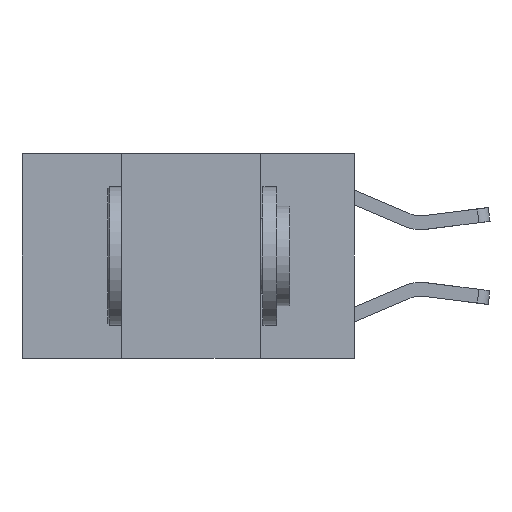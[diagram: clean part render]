
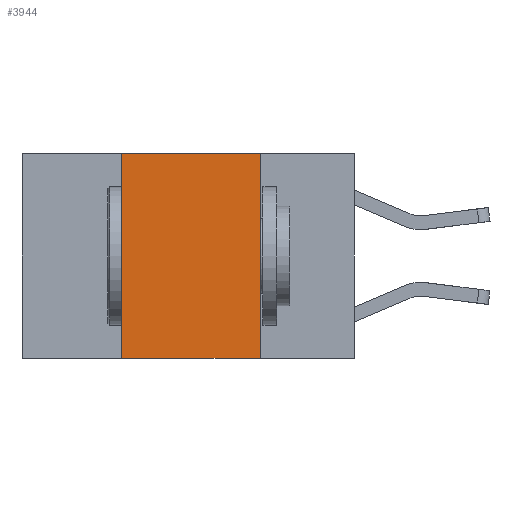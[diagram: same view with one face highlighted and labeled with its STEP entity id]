
A CAD part, left-side view. The second image highlights one B-rep face of the part: STEP entity #3944.
In plain terms, the highlighted planar face has unit normal (-1, 0, 0).
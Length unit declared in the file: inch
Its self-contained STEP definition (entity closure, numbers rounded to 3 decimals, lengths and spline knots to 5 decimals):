
#941 = AXIS2_PLACEMENT_3D ( 'NONE', #8948, #4340, #2792 ) ;
#1291 = ORIENTED_EDGE ( 'NONE', *, *, #2422, .F. ) ;
#1831 = DIRECTION ( 'NONE',  ( 0., 0., -1. ) ) ;
#1952 = ORIENTED_EDGE ( 'NONE', *, *, #6534, .F. ) ;
#2422 = EDGE_CURVE ( 'NONE', #3168, #3902, #9330, .T. ) ;
#2683 = VECTOR ( 'NONE', #4511, 39.37008 ) ;
#2792 = DIRECTION ( 'NONE',  ( 0., 0., -1. ) ) ;
#3014 = CARTESIAN_POINT ( 'NONE',  ( 0., 0.6, 0. ) ) ;
#3054 = LINE ( 'NONE', #8457, #4012 ) ;
#3105 = DIRECTION ( 'NONE',  ( 0., -1., 0. ) ) ;
#3168 = VERTEX_POINT ( 'NONE', #9016 ) ;
#3564 = VECTOR ( 'NONE', #4637, 39.37008 ) ;
#3902 = VERTEX_POINT ( 'NONE', #9345 ) ;
#3944 = ADVANCED_FACE ( 'NONE', ( #5089 ), #9685, .F. ) ;
#4012 = VECTOR ( 'NONE', #3105, 39.37008 ) ;
#4340 = DIRECTION ( 'NONE',  ( 1., 0., 0. ) ) ;
#4456 = VERTEX_POINT ( 'NONE', #6761 ) ;
#4511 = DIRECTION ( 'NONE',  ( 0., -1., 0. ) ) ;
#4637 = DIRECTION ( 'NONE',  ( 0., 0., 1. ) ) ;
#4737 = CARTESIAN_POINT ( 'NONE',  ( 0., 0.42, 0. ) ) ;
#4993 = EDGE_CURVE ( 'NONE', #3168, #7011, #3054, .T. ) ;
#5089 = FACE_OUTER_BOUND ( 'NONE', #5743, .T. ) ;
#5211 = ORIENTED_EDGE ( 'NONE', *, *, #9650, .F. ) ;
#5688 = CARTESIAN_POINT ( 'NONE',  ( 0., 0.17, 0. ) ) ;
#5743 = EDGE_LOOP ( 'NONE', ( #5211, #1952, #1291, #8665 ) ) ;
#6534 = EDGE_CURVE ( 'NONE', #3902, #4456, #9758, .T. ) ;
#6761 = CARTESIAN_POINT ( 'NONE',  ( 0., 0.17, 0. ) ) ;
#7011 = VERTEX_POINT ( 'NONE', #7456 ) ;
#7028 = VECTOR ( 'NONE', #1831, 39.37008 ) ;
#7456 = CARTESIAN_POINT ( 'NONE',  ( 0., 0.17, -0.37 ) ) ;
#7770 = LINE ( 'NONE', #5688, #7028 ) ;
#8457 = CARTESIAN_POINT ( 'NONE',  ( 0., 0.6, -0.37 ) ) ;
#8665 = ORIENTED_EDGE ( 'NONE', *, *, #4993, .T. ) ;
#8948 = CARTESIAN_POINT ( 'NONE',  ( 0., 0.6, 0. ) ) ;
#9016 = CARTESIAN_POINT ( 'NONE',  ( 0., 0.42, -0.37 ) ) ;
#9330 = LINE ( 'NONE', #4737, #3564 ) ;
#9345 = CARTESIAN_POINT ( 'NONE',  ( 0., 0.42, 0. ) ) ;
#9650 = EDGE_CURVE ( 'NONE', #4456, #7011, #7770, .T. ) ;
#9685 = PLANE ( 'NONE',  #941 ) ;
#9758 = LINE ( 'NONE', #3014, #2683 ) ;
